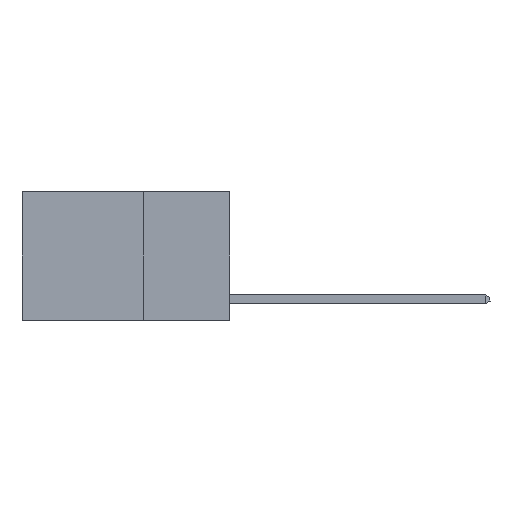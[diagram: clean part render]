
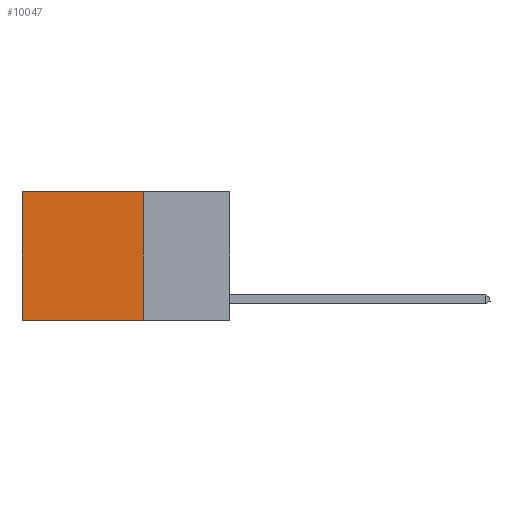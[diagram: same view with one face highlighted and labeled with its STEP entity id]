
A CAD part, left-side view. The second image highlights one B-rep face of the part: STEP entity #10047.
In plain terms, the highlighted planar face has unit normal (-1, 0, 0).
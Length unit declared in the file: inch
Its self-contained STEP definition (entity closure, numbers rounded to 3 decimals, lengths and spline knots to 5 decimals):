
#460 = LINE ( 'NONE', #550, #709 ) ;
#550 = CARTESIAN_POINT ( 'NONE',  ( 0.2625, 0.25, 0. ) ) ;
#709 = VECTOR ( 'NONE', #14661, 39.37008 ) ;
#762 = ORIENTED_EDGE ( 'NONE', *, *, #3912, .F. ) ;
#1760 = LINE ( 'NONE', #3225, #13648 ) ;
#2991 = ORIENTED_EDGE ( 'NONE', *, *, #16494, .F. ) ;
#3225 = CARTESIAN_POINT ( 'NONE',  ( 0.2625, 0.25, 0. ) ) ;
#3912 = EDGE_CURVE ( 'NONE', #15358, #8075, #460, .T. ) ;
#4274 = CARTESIAN_POINT ( 'NONE',  ( 0.2625, 0.6, 0. ) ) ;
#5184 = ORIENTED_EDGE ( 'NONE', *, *, #17002, .T. ) ;
#5218 = DIRECTION ( 'NONE',  ( 0., 0., -1. ) ) ;
#5820 = VERTEX_POINT ( 'NONE', #4274 ) ;
#6325 = VECTOR ( 'NONE', #10971, 39.37008 ) ;
#6805 = ORIENTED_EDGE ( 'NONE', *, *, #13675, .T. ) ;
#7205 = VECTOR ( 'NONE', #15050, 39.37008 ) ;
#7239 = CARTESIAN_POINT ( 'NONE',  ( 0.2625, 0.6, -0.37 ) ) ;
#8040 = CARTESIAN_POINT ( 'NONE',  ( 0.2625, 0.25, -0.37 ) ) ;
#8075 = VERTEX_POINT ( 'NONE', #12006 ) ;
#8089 = CARTESIAN_POINT ( 'NONE',  ( 0.2625, 0.25, 0. ) ) ;
#9444 = LINE ( 'NONE', #8040, #7205 ) ;
#10047 = ADVANCED_FACE ( 'NONE', ( #12250 ), #17877, .F. ) ;
#10053 = AXIS2_PLACEMENT_3D ( 'NONE', #8089, #11042, #5218 ) ;
#10079 = CARTESIAN_POINT ( 'NONE',  ( 0.2625, 0.25, 0. ) ) ;
#10710 = CARTESIAN_POINT ( 'NONE',  ( 0.2625, 0.6, 0. ) ) ;
#10971 = DIRECTION ( 'NONE',  ( 0., 0., -1. ) ) ;
#11042 = DIRECTION ( 'NONE',  ( 1., 0., 0. ) ) ;
#12006 = CARTESIAN_POINT ( 'NONE',  ( 0.2625, 0.25, -0.37 ) ) ;
#12250 = FACE_OUTER_BOUND ( 'NONE', #17078, .T. ) ;
#13648 = VECTOR ( 'NONE', #17462, 39.37008 ) ;
#13675 = EDGE_CURVE ( 'NONE', #15358, #5820, #1760, .T. ) ;
#14520 = VERTEX_POINT ( 'NONE', #7239 ) ;
#14661 = DIRECTION ( 'NONE',  ( 0., 0., -1. ) ) ;
#15050 = DIRECTION ( 'NONE',  ( 0., 1., 0. ) ) ;
#15358 = VERTEX_POINT ( 'NONE', #10079 ) ;
#16494 = EDGE_CURVE ( 'NONE', #8075, #14520, #9444, .T. ) ;
#17002 = EDGE_CURVE ( 'NONE', #5820, #14520, #17897, .T. ) ;
#17078 = EDGE_LOOP ( 'NONE', ( #5184, #2991, #762, #6805 ) ) ;
#17462 = DIRECTION ( 'NONE',  ( 0., 1., 0. ) ) ;
#17877 = PLANE ( 'NONE',  #10053 ) ;
#17897 = LINE ( 'NONE', #10710, #6325 ) ;
